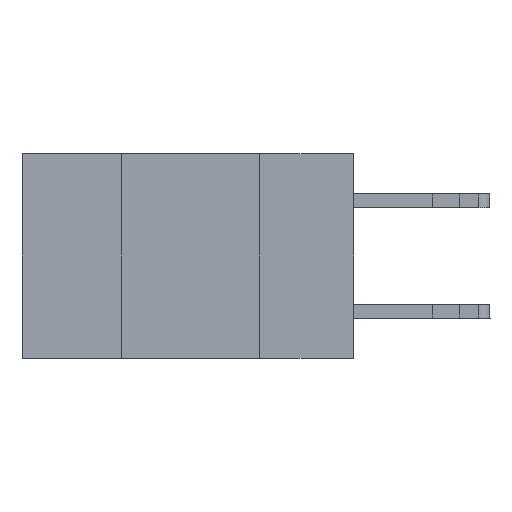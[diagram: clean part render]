
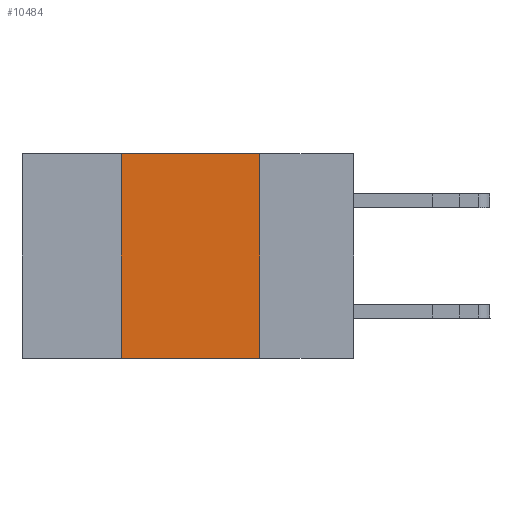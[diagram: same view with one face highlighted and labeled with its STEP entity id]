
A CAD part, left-side view. The second image highlights one B-rep face of the part: STEP entity #10484.
In plain terms, the highlighted planar face has unit normal (-1, 0, 0).
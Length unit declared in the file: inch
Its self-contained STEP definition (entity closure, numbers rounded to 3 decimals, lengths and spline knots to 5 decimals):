
#1433 = VECTOR ( 'NONE', #15414, 39.37008 ) ;
#1447 = FACE_OUTER_BOUND ( 'NONE', #5921, .T. ) ;
#1532 = DIRECTION ( 'NONE',  ( 1., 0., 0. ) ) ;
#1957 = LINE ( 'NONE', #15022, #12678 ) ;
#3607 = ORIENTED_EDGE ( 'NONE', *, *, #14347, .F. ) ;
#3805 = CARTESIAN_POINT ( 'NONE',  ( 0., 0.42, 0. ) ) ;
#3900 = VERTEX_POINT ( 'NONE', #7299 ) ;
#4587 = EDGE_CURVE ( 'NONE', #11181, #8001, #1957, .T. ) ;
#4700 = ORIENTED_EDGE ( 'NONE', *, *, #6258, .T. ) ;
#4783 = LINE ( 'NONE', #7367, #13191 ) ;
#5921 = EDGE_LOOP ( 'NONE', ( #16035, #3607, #16140, #4700 ) ) ;
#6258 = EDGE_CURVE ( 'NONE', #7317, #8001, #4783, .T. ) ;
#7040 = CARTESIAN_POINT ( 'NONE',  ( 0., 0.17, 0. ) ) ;
#7079 = DIRECTION ( 'NONE',  ( 0., 0., -1. ) ) ;
#7299 = CARTESIAN_POINT ( 'NONE',  ( 0., 0.42, 0. ) ) ;
#7317 = VERTEX_POINT ( 'NONE', #11101 ) ;
#7361 = EDGE_CURVE ( 'NONE', #7317, #3900, #8523, .T. ) ;
#7367 = CARTESIAN_POINT ( 'NONE',  ( 0., 0.6, -0.37 ) ) ;
#7463 = DIRECTION ( 'NONE',  ( 0., -1., 0. ) ) ;
#7666 = CARTESIAN_POINT ( 'NONE',  ( 0., 0.6, 0. ) ) ;
#8001 = VERTEX_POINT ( 'NONE', #11127 ) ;
#8523 = LINE ( 'NONE', #3805, #14777 ) ;
#9194 = LINE ( 'NONE', #7666, #1433 ) ;
#9299 = PLANE ( 'NONE',  #15400 ) ;
#9375 = DIRECTION ( 'NONE',  ( 0., 0., -1. ) ) ;
#10484 = ADVANCED_FACE ( 'NONE', ( #1447 ), #9299, .F. ) ;
#11101 = CARTESIAN_POINT ( 'NONE',  ( 0., 0.42, -0.37 ) ) ;
#11127 = CARTESIAN_POINT ( 'NONE',  ( 0., 0.17, -0.37 ) ) ;
#11181 = VERTEX_POINT ( 'NONE', #7040 ) ;
#12539 = DIRECTION ( 'NONE',  ( 0., 0., 1. ) ) ;
#12678 = VECTOR ( 'NONE', #7079, 39.37008 ) ;
#13191 = VECTOR ( 'NONE', #7463, 39.37008 ) ;
#14347 = EDGE_CURVE ( 'NONE', #3900, #11181, #9194, .T. ) ;
#14438 = CARTESIAN_POINT ( 'NONE',  ( 0., 0.6, 0. ) ) ;
#14777 = VECTOR ( 'NONE', #12539, 39.37008 ) ;
#15022 = CARTESIAN_POINT ( 'NONE',  ( 0., 0.17, 0. ) ) ;
#15400 = AXIS2_PLACEMENT_3D ( 'NONE', #14438, #1532, #9375 ) ;
#15414 = DIRECTION ( 'NONE',  ( 0., -1., 0. ) ) ;
#16035 = ORIENTED_EDGE ( 'NONE', *, *, #4587, .F. ) ;
#16140 = ORIENTED_EDGE ( 'NONE', *, *, #7361, .F. ) ;
